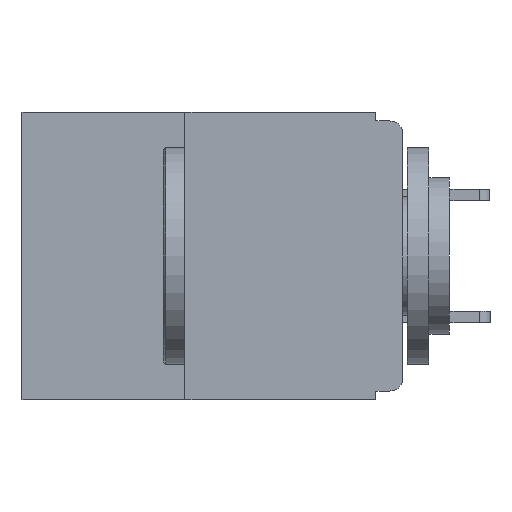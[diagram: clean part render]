
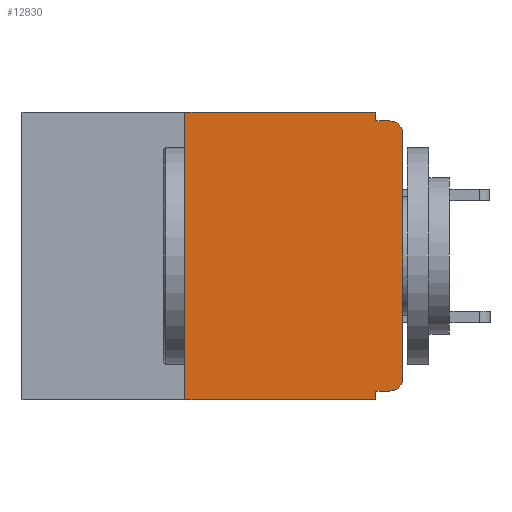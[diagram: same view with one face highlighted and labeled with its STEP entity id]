
A CAD part, left-side view. The second image highlights one B-rep face of the part: STEP entity #12830.
In plain terms, the highlighted planar face has unit normal (-1, 0, 0).
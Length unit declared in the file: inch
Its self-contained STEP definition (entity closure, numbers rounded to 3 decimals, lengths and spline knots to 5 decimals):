
#496 = DIRECTION ( 'NONE',  ( 0., -1., 0. ) ) ;
#497 = CARTESIAN_POINT ( 'NONE',  ( 0., 0.015, -0.01 ) ) ;
#512 = DIRECTION ( 'NONE',  ( 0., 0., 1. ) ) ;
#828 = AXIS2_PLACEMENT_3D ( 'NONE', #16830, #2177, #19289 ) ;
#1016 = VERTEX_POINT ( 'NONE', #18477 ) ;
#1174 = CARTESIAN_POINT ( 'NONE',  ( 0., 0.437, 0. ) ) ;
#1227 = EDGE_CURVE ( 'NONE', #10187, #17891, #13382, .T. ) ;
#1881 = VECTOR ( 'NONE', #512, 39.37008 ) ;
#2130 = VERTEX_POINT ( 'NONE', #26783 ) ;
#2177 = DIRECTION ( 'NONE',  ( -1., 0., 0. ) ) ;
#2538 = EDGE_CURVE ( 'NONE', #14176, #28321, #19003, .T. ) ;
#2600 = ORIENTED_EDGE ( 'NONE', *, *, #23881, .T. ) ;
#3010 = ORIENTED_EDGE ( 'NONE', *, *, #7999, .F. ) ;
#3051 = CARTESIAN_POINT ( 'NONE',  ( 0., 0.25, -0.33 ) ) ;
#3726 = CARTESIAN_POINT ( 'NONE',  ( 0., 0.031, -0.01 ) ) ;
#3849 = VERTEX_POINT ( 'NONE', #27288 ) ;
#4595 = EDGE_LOOP ( 'NONE', ( #2600, #9022, #9774, #29261, #11335, #30700, #7125, #15261, #3010, #9419 ) ) ;
#5256 = VERTEX_POINT ( 'NONE', #15242 ) ;
#5327 = VECTOR ( 'NONE', #15099, 39.37008 ) ;
#6837 = DIRECTION ( 'NONE',  ( 0., 1., 0. ) ) ;
#6893 = CARTESIAN_POINT ( 'NONE',  ( 0., 0.015, -0.025 ) ) ;
#7125 = ORIENTED_EDGE ( 'NONE', *, *, #1227, .T. ) ;
#7694 = CARTESIAN_POINT ( 'NONE',  ( 0., 0., -0.01 ) ) ;
#7999 = EDGE_CURVE ( 'NONE', #11388, #3849, #30067, .T. ) ;
#8204 = CARTESIAN_POINT ( 'NONE',  ( 0., 0.031, -0.33 ) ) ;
#8614 = LINE ( 'NONE', #21935, #14404 ) ;
#9019 = CIRCLE ( 'NONE', #29825, 0.015 ) ;
#9022 = ORIENTED_EDGE ( 'NONE', *, *, #29829, .T. ) ;
#9320 = LINE ( 'NONE', #28871, #21699 ) ;
#9334 = DIRECTION ( 'NONE',  ( 0., 0., -1. ) ) ;
#9419 = ORIENTED_EDGE ( 'NONE', *, *, #18501, .T. ) ;
#9774 = ORIENTED_EDGE ( 'NONE', *, *, #2538, .F. ) ;
#10187 = VERTEX_POINT ( 'NONE', #3051 ) ;
#10827 = CARTESIAN_POINT ( 'NONE',  ( 0., 0., -0.305 ) ) ;
#10934 = DIRECTION ( 'NONE',  ( 0., 0., -1. ) ) ;
#11031 = AXIS2_PLACEMENT_3D ( 'NONE', #1174, #25660, #10934 ) ;
#11335 = ORIENTED_EDGE ( 'NONE', *, *, #17321, .F. ) ;
#11388 = VERTEX_POINT ( 'NONE', #17174 ) ;
#12209 = VECTOR ( 'NONE', #6837, 39.37008 ) ;
#12320 = CARTESIAN_POINT ( 'NONE',  ( 0., 0., -0.32 ) ) ;
#12606 = CARTESIAN_POINT ( 'NONE',  ( 0., 0., 0. ) ) ;
#12682 = EDGE_CURVE ( 'NONE', #10187, #5256, #27852, .T. ) ;
#12830 = ADVANCED_FACE ( 'NONE', ( #28950 ), #23272, .F. ) ;
#13382 = LINE ( 'NONE', #25427, #31105 ) ;
#14176 = VERTEX_POINT ( 'NONE', #3726 ) ;
#14404 = VECTOR ( 'NONE', #29043, 39.37008 ) ;
#15099 = DIRECTION ( 'NONE',  ( 0., 0., 1. ) ) ;
#15242 = CARTESIAN_POINT ( 'NONE',  ( 0., 0.25, 0. ) ) ;
#15261 = ORIENTED_EDGE ( 'NONE', *, *, #29562, .F. ) ;
#16830 = CARTESIAN_POINT ( 'NONE',  ( 0., 0.015, -0.305 ) ) ;
#17174 = CARTESIAN_POINT ( 'NONE',  ( 0., 0.015, -0.32 ) ) ;
#17321 = EDGE_CURVE ( 'NONE', #5256, #1016, #9320, .T. ) ;
#17891 = VERTEX_POINT ( 'NONE', #29054 ) ;
#18477 = CARTESIAN_POINT ( 'NONE',  ( 0., 0.031, 0. ) ) ;
#18501 = EDGE_CURVE ( 'NONE', #11388, #20314, #20439, .T. ) ;
#19003 = LINE ( 'NONE', #7694, #31017 ) ;
#19289 = DIRECTION ( 'NONE',  ( 0., 0., -1. ) ) ;
#20314 = VERTEX_POINT ( 'NONE', #10827 ) ;
#20439 = CIRCLE ( 'NONE', #828, 0.015 ) ;
#21699 = VECTOR ( 'NONE', #31179, 39.37008 ) ;
#21935 = CARTESIAN_POINT ( 'NONE',  ( 0., 0.031, 0. ) ) ;
#22510 = DIRECTION ( 'NONE',  ( 0., -1., 0. ) ) ;
#22607 = EDGE_CURVE ( 'NONE', #1016, #14176, #8614, .T. ) ;
#22635 = CARTESIAN_POINT ( 'NONE',  ( 0., 0.25, -0.33 ) ) ;
#23272 = PLANE ( 'NONE',  #11031 ) ;
#23881 = EDGE_CURVE ( 'NONE', #20314, #2130, #24880, .T. ) ;
#24104 = DIRECTION ( 'NONE',  ( -1., 0., 0. ) ) ;
#24880 = LINE ( 'NONE', #12606, #5327 ) ;
#24919 = LINE ( 'NONE', #8204, #30447 ) ;
#25427 = CARTESIAN_POINT ( 'NONE',  ( 0., 0.437, -0.33 ) ) ;
#25660 = DIRECTION ( 'NONE',  ( 1., 0., 0. ) ) ;
#26783 = CARTESIAN_POINT ( 'NONE',  ( 0., 0., -0.025 ) ) ;
#27288 = CARTESIAN_POINT ( 'NONE',  ( 0., 0.031, -0.32 ) ) ;
#27772 = DIRECTION ( 'NONE',  ( 0., 0., -1. ) ) ;
#27852 = LINE ( 'NONE', #22635, #1881 ) ;
#28321 = VERTEX_POINT ( 'NONE', #497 ) ;
#28871 = CARTESIAN_POINT ( 'NONE',  ( 0., 0.437, 0. ) ) ;
#28950 = FACE_OUTER_BOUND ( 'NONE', #4595, .T. ) ;
#29043 = DIRECTION ( 'NONE',  ( 0., 0., -1. ) ) ;
#29054 = CARTESIAN_POINT ( 'NONE',  ( 0., 0.031, -0.33 ) ) ;
#29261 = ORIENTED_EDGE ( 'NONE', *, *, #22607, .F. ) ;
#29562 = EDGE_CURVE ( 'NONE', #3849, #17891, #24919, .T. ) ;
#29825 = AXIS2_PLACEMENT_3D ( 'NONE', #6893, #24104, #9334 ) ;
#29829 = EDGE_CURVE ( 'NONE', #2130, #28321, #9019, .T. ) ;
#30067 = LINE ( 'NONE', #12320, #12209 ) ;
#30447 = VECTOR ( 'NONE', #27772, 39.37008 ) ;
#30700 = ORIENTED_EDGE ( 'NONE', *, *, #12682, .F. ) ;
#31017 = VECTOR ( 'NONE', #496, 39.37008 ) ;
#31105 = VECTOR ( 'NONE', #22510, 39.37008 ) ;
#31179 = DIRECTION ( 'NONE',  ( 0., -1., 0. ) ) ;
